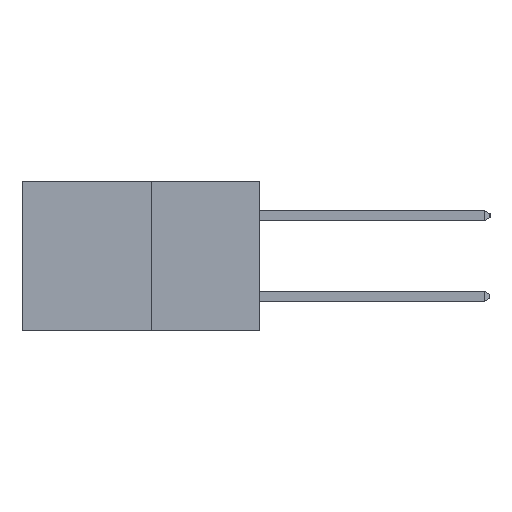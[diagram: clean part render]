
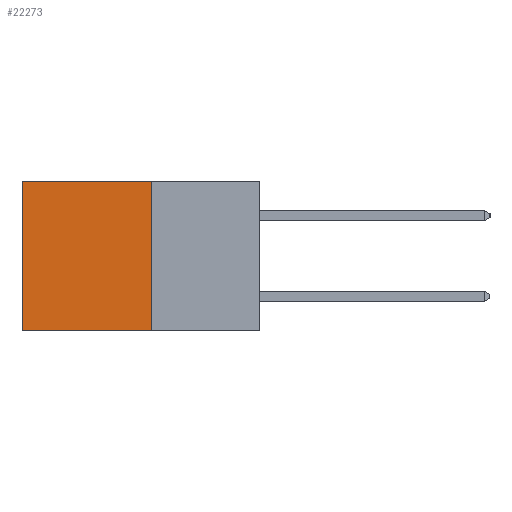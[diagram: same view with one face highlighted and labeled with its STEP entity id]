
A CAD part, left-side view. The second image highlights one B-rep face of the part: STEP entity #22273.
In plain terms, the highlighted planar face has unit normal (-1, 0, 0).
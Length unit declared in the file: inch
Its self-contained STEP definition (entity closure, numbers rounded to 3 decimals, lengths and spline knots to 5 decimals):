
#1183 = PLANE ( 'NONE',  #1202 ) ;
#1202 = AXIS2_PLACEMENT_3D ( 'NONE', #20127, #8958, #21972 ) ;
#1994 = CARTESIAN_POINT ( 'NONE',  ( 0.277, 0.27, -0.37 ) ) ;
#3306 = FACE_OUTER_BOUND ( 'NONE', #16224, .T. ) ;
#3727 = LINE ( 'NONE', #22208, #9483 ) ;
#3742 = CARTESIAN_POINT ( 'NONE',  ( 0.277, 0.27, -0.37 ) ) ;
#4163 = CARTESIAN_POINT ( 'NONE',  ( 0.277, 0.59, -0.37 ) ) ;
#4203 = EDGE_CURVE ( 'NONE', #12118, #14855, #6171, .T. ) ;
#5494 = VECTOR ( 'NONE', #15388, 39.37008 ) ;
#5926 = VERTEX_POINT ( 'NONE', #4163 ) ;
#6171 = LINE ( 'NONE', #11587, #11278 ) ;
#6783 = CARTESIAN_POINT ( 'NONE',  ( 0.277, 0.27, 0. ) ) ;
#7364 = ORIENTED_EDGE ( 'NONE', *, *, #20285, .T. ) ;
#8958 = DIRECTION ( 'NONE',  ( 1., 0., 0. ) ) ;
#9483 = VECTOR ( 'NONE', #16594, 39.37008 ) ;
#10620 = LINE ( 'NONE', #1994, #5494 ) ;
#11278 = VECTOR ( 'NONE', #17758, 39.37008 ) ;
#11587 = CARTESIAN_POINT ( 'NONE',  ( 0.277, 0.27, 0. ) ) ;
#12118 = VERTEX_POINT ( 'NONE', #6783 ) ;
#13495 = ORIENTED_EDGE ( 'NONE', *, *, #17800, .F. ) ;
#14855 = VERTEX_POINT ( 'NONE', #21079 ) ;
#15128 = DIRECTION ( 'NONE',  ( 0., 1., 0. ) ) ;
#15388 = DIRECTION ( 'NONE',  ( 0., 0., -1. ) ) ;
#16224 = EDGE_LOOP ( 'NONE', ( #7364, #13495, #21684, #16639 ) ) ;
#16594 = DIRECTION ( 'NONE',  ( 0., 0., -1. ) ) ;
#16639 = ORIENTED_EDGE ( 'NONE', *, *, #4203, .T. ) ;
#16904 = CARTESIAN_POINT ( 'NONE',  ( 0.277, 0.27, -0.37 ) ) ;
#17758 = DIRECTION ( 'NONE',  ( 0., 1., 0. ) ) ;
#17800 = EDGE_CURVE ( 'NONE', #20387, #5926, #23758, .T. ) ;
#18275 = VECTOR ( 'NONE', #15128, 39.37008 ) ;
#20127 = CARTESIAN_POINT ( 'NONE',  ( 0.277, 0.27, -0.37 ) ) ;
#20285 = EDGE_CURVE ( 'NONE', #14855, #5926, #3727, .T. ) ;
#20387 = VERTEX_POINT ( 'NONE', #16904 ) ;
#21068 = EDGE_CURVE ( 'NONE', #12118, #20387, #10620, .T. ) ;
#21079 = CARTESIAN_POINT ( 'NONE',  ( 0.277, 0.59, 0. ) ) ;
#21684 = ORIENTED_EDGE ( 'NONE', *, *, #21068, .F. ) ;
#21972 = DIRECTION ( 'NONE',  ( 0., 0., -1. ) ) ;
#22208 = CARTESIAN_POINT ( 'NONE',  ( 0.277, 0.59, -0.37 ) ) ;
#22273 = ADVANCED_FACE ( 'NONE', ( #3306 ), #1183, .F. ) ;
#23758 = LINE ( 'NONE', #3742, #18275 ) ;
